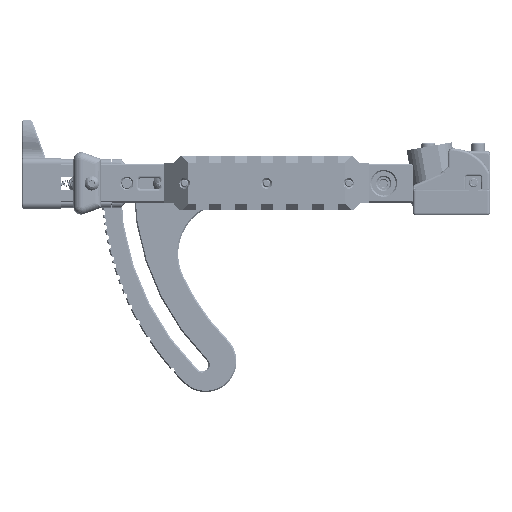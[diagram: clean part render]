
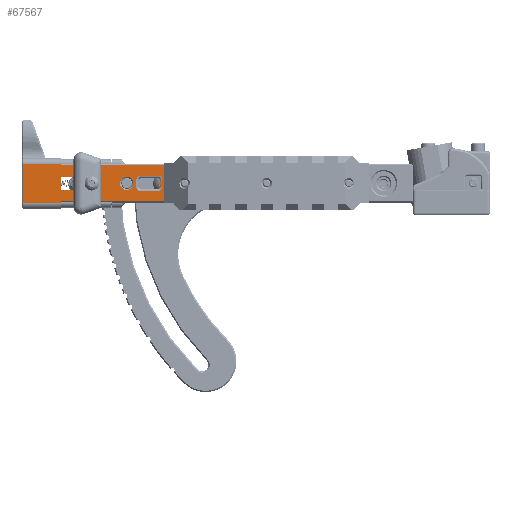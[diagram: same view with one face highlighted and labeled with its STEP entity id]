
A CAD part, left-side view. The second image highlights one B-rep face of the part: STEP entity #67567.
In plain terms, the highlighted planar face has unit normal (-1, 0, 0).
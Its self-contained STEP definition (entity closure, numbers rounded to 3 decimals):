
#2247=FACE_BOUND('',#20366,.T.);
#2248=FACE_BOUND('',#20367,.T.);
#2249=FACE_BOUND('',#20368,.T.);
#3197=PLANE('',#73201);
#6426=LINE('',#202842,#10051);
#6439=LINE('',#202868,#10064);
#6453=LINE('',#202906,#10078);
#6454=LINE('',#202908,#10079);
#6455=LINE('',#202910,#10080);
#6456=LINE('',#202912,#10081);
#6457=LINE('',#202914,#10082);
#6458=LINE('',#202915,#10083);
#6459=LINE('',#202918,#10084);
#6460=LINE('',#202920,#10085);
#6461=LINE('',#202922,#10086);
#6462=LINE('',#202923,#10087);
#6463=LINE('',#202928,#10088);
#6464=LINE('',#202930,#10089);
#6465=LINE('',#202932,#10090);
#6466=LINE('',#202936,#10091);
#6467=LINE('',#202940,#10092);
#6468=LINE('',#202944,#10093);
#6469=LINE('',#202947,#10094);
#10051=VECTOR('',#86486,10.);
#10064=VECTOR('',#86507,10.);
#10078=VECTOR('',#86529,10.);
#10079=VECTOR('',#86530,10.);
#10080=VECTOR('',#86531,10.);
#10081=VECTOR('',#86532,10.);
#10082=VECTOR('',#86533,10.);
#10083=VECTOR('',#86534,10.);
#10084=VECTOR('',#86535,10.);
#10085=VECTOR('',#86536,10.);
#10086=VECTOR('',#86537,10.);
#10087=VECTOR('',#86538,10.);
#10088=VECTOR('',#86541,10.);
#10089=VECTOR('',#86542,10.);
#10090=VECTOR('',#86543,10.);
#10091=VECTOR('',#86546,10.);
#10092=VECTOR('',#86549,10.);
#10093=VECTOR('',#86552,10.);
#10094=VECTOR('',#86555,10.);
#16200=FACE_OUTER_BOUND('',#20365,.T.);
#20365=EDGE_LOOP('',(#60392,#60393,#60394,#60395,#60396,#60397,#60398,#60399));
#20366=EDGE_LOOP('',(#60400,#60401,#60402,#60403));
#20367=EDGE_LOOP('',(#60404));
#20368=EDGE_LOOP('',(#60405,#60406,#60407,#60408,#60409,#60410,#60411,#60412,
#60413,#60414,#60415));
#22561=CIRCLE('',#73202,2.6);
#22562=CIRCLE('',#73203,1.5);
#22563=CIRCLE('',#73204,1.5);
#22564=CIRCLE('',#73205,1.5);
#22565=CIRCLE('',#73206,1.5);
#31905=VERTEX_POINT('',#202839);
#31906=VERTEX_POINT('',#202841);
#31915=VERTEX_POINT('',#202867);
#31928=VERTEX_POINT('',#202905);
#31929=VERTEX_POINT('',#202907);
#31930=VERTEX_POINT('',#202909);
#31931=VERTEX_POINT('',#202911);
#31932=VERTEX_POINT('',#202913);
#31933=VERTEX_POINT('',#202916);
#31934=VERTEX_POINT('',#202917);
#31935=VERTEX_POINT('',#202919);
#31936=VERTEX_POINT('',#202921);
#31937=VERTEX_POINT('',#202924);
#31938=VERTEX_POINT('',#202926);
#31939=VERTEX_POINT('',#202927);
#31940=VERTEX_POINT('',#202929);
#31941=VERTEX_POINT('',#202931);
#31942=VERTEX_POINT('',#202933);
#31943=VERTEX_POINT('',#202935);
#31944=VERTEX_POINT('',#202937);
#31945=VERTEX_POINT('',#202939);
#31946=VERTEX_POINT('',#202941);
#31947=VERTEX_POINT('',#202943);
#31948=VERTEX_POINT('',#202945);
#41588=EDGE_CURVE('',#31906,#31905,#6426,.T.);
#41601=EDGE_CURVE('',#31906,#31915,#6439,.T.);
#41617=EDGE_CURVE('',#31928,#31905,#6453,.T.);
#41618=EDGE_CURVE('',#31929,#31928,#6454,.T.);
#41619=EDGE_CURVE('',#31929,#31930,#6455,.T.);
#41620=EDGE_CURVE('',#31931,#31930,#6456,.T.);
#41621=EDGE_CURVE('',#31931,#31932,#6457,.T.);
#41622=EDGE_CURVE('',#31915,#31932,#6458,.T.);
#41623=EDGE_CURVE('',#31933,#31934,#6459,.T.);
#41624=EDGE_CURVE('',#31935,#31933,#6460,.T.);
#41625=EDGE_CURVE('',#31936,#31935,#6461,.T.);
#41626=EDGE_CURVE('',#31934,#31936,#6462,.T.);
#41627=EDGE_CURVE('',#31937,#31937,#22561,.T.);
#41628=EDGE_CURVE('',#31938,#31939,#6463,.T.);
#41629=EDGE_CURVE('',#31939,#31940,#6464,.T.);
#41630=EDGE_CURVE('',#31941,#31940,#6465,.T.);
#41631=EDGE_CURVE('',#31942,#31941,#22562,.T.);
#41632=EDGE_CURVE('',#31943,#31942,#6466,.T.);
#41633=EDGE_CURVE('',#31944,#31943,#22563,.T.);
#41634=EDGE_CURVE('',#31945,#31944,#6467,.T.);
#41635=EDGE_CURVE('',#31946,#31945,#22564,.T.);
#41636=EDGE_CURVE('',#31947,#31946,#6468,.T.);
#41637=EDGE_CURVE('',#31948,#31947,#22565,.T.);
#41638=EDGE_CURVE('',#31938,#31948,#6469,.T.);
#60392=ORIENTED_EDGE('',*,*,#41588,.T.);
#60393=ORIENTED_EDGE('',*,*,#41617,.F.);
#60394=ORIENTED_EDGE('',*,*,#41618,.F.);
#60395=ORIENTED_EDGE('',*,*,#41619,.T.);
#60396=ORIENTED_EDGE('',*,*,#41620,.F.);
#60397=ORIENTED_EDGE('',*,*,#41621,.T.);
#60398=ORIENTED_EDGE('',*,*,#41622,.F.);
#60399=ORIENTED_EDGE('',*,*,#41601,.F.);
#60400=ORIENTED_EDGE('',*,*,#41623,.F.);
#60401=ORIENTED_EDGE('',*,*,#41624,.F.);
#60402=ORIENTED_EDGE('',*,*,#41625,.F.);
#60403=ORIENTED_EDGE('',*,*,#41626,.F.);
#60404=ORIENTED_EDGE('',*,*,#41627,.F.);
#60405=ORIENTED_EDGE('',*,*,#41628,.T.);
#60406=ORIENTED_EDGE('',*,*,#41629,.T.);
#60407=ORIENTED_EDGE('',*,*,#41630,.F.);
#60408=ORIENTED_EDGE('',*,*,#41631,.F.);
#60409=ORIENTED_EDGE('',*,*,#41632,.F.);
#60410=ORIENTED_EDGE('',*,*,#41633,.F.);
#60411=ORIENTED_EDGE('',*,*,#41634,.F.);
#60412=ORIENTED_EDGE('',*,*,#41635,.F.);
#60413=ORIENTED_EDGE('',*,*,#41636,.F.);
#60414=ORIENTED_EDGE('',*,*,#41637,.F.);
#60415=ORIENTED_EDGE('',*,*,#41638,.F.);
#67567=ADVANCED_FACE('',(#16200,#2247,#2248,#2249),#3197,.T.);
#73201=AXIS2_PLACEMENT_3D('',#202904,#86527,#86528);
#73202=AXIS2_PLACEMENT_3D('',#202925,#86539,#86540);
#73203=AXIS2_PLACEMENT_3D('',#202934,#86544,#86545);
#73204=AXIS2_PLACEMENT_3D('',#202938,#86547,#86548);
#73205=AXIS2_PLACEMENT_3D('',#202942,#86550,#86551);
#73206=AXIS2_PLACEMENT_3D('',#202946,#86553,#86554);
#86486=DIRECTION('',(0.,0.,1.));
#86507=DIRECTION('',(0.,1.,0.));
#86527=DIRECTION('center_axis',(-1.,0.,
0.));
#86528=DIRECTION('ref_axis',(0.,0.,
1.));
#86529=DIRECTION('',(0.,-1.,0.));
#86530=DIRECTION('',(0.,0.,-1.));
#86531=DIRECTION('',(0.,1.,0.));
#86532=DIRECTION('',(0.,0.,1.));
#86533=DIRECTION('',(0.,-1.,0.));
#86534=DIRECTION('',(0.,0.,-1.));
#86535=DIRECTION('',(0.,0.,-1.));
#86536=DIRECTION('',(0.,1.,0.));
#86537=DIRECTION('',(0.,0.,1.));
#86538=DIRECTION('',(0.,-1.,0.));
#86539=DIRECTION('center_axis',(-1.,0.,
0.));
#86540=DIRECTION('ref_axis',(0.,0.,
1.));
#86541=DIRECTION('',(0.,0.866,-0.5));
#86542=DIRECTION('',(0.,-0.866,-0.5));
#86543=DIRECTION('',(0.,0.,1.));
#86544=DIRECTION('center_axis',(-1.,0.,
0.));
#86545=DIRECTION('ref_axis',(0.,-0.707,-0.707));
#86546=DIRECTION('',(0.,-1.,0.));
#86547=DIRECTION('center_axis',(-1.,0.,
0.));
#86548=DIRECTION('ref_axis',(0.,0.707,-0.707));
#86549=DIRECTION('',(0.,0.,-1.));
#86550=DIRECTION('center_axis',(-1.,0.,
0.));
#86551=DIRECTION('ref_axis',(0.,0.707,0.707));
#86552=DIRECTION('',(0.,1.,0.));
#86553=DIRECTION('center_axis',(-1.,0.,
0.));
#86554=DIRECTION('ref_axis',(0.,-0.707,0.707));
#86555=DIRECTION('',(0.,0.,1.));
#202839=CARTESIAN_POINT('',(-55.716,-306.888,31.511));
#202841=CARTESIAN_POINT('',(-55.716,-306.888,17.511));
#202842=CARTESIAN_POINT('',(-55.716,-306.888,20.476));
#202867=CARTESIAN_POINT('',(-55.71,-266.641,17.511));
#202868=CARTESIAN_POINT('',(-55.713,-289.093,17.511));
#202904=CARTESIAN_POINT('Origin',(-55.719,-326.593,24.511));
#202905=CARTESIAN_POINT('',(-55.71,-266.641,31.511));
#202906=CARTESIAN_POINT('',(-55.725,-364.093,31.511));
#202907=CARTESIAN_POINT('',(-55.71,-266.641,32.011));
#202908=CARTESIAN_POINT('',(-55.71,-266.641,24.511));
#202909=CARTESIAN_POINT('',(-55.707,-252.094,32.011));
#202910=CARTESIAN_POINT('',(-55.71,-266.641,32.011));
#202911=CARTESIAN_POINT('',(-55.707,-252.094,17.011));
#202912=CARTESIAN_POINT('',(-55.707,-252.094,19.511));
#202913=CARTESIAN_POINT('',(-55.71,-266.641,17.011));
#202914=CARTESIAN_POINT('',(-55.731,-401.593,17.011));
#202915=CARTESIAN_POINT('',(-55.71,-266.641,24.511));
#202916=CARTESIAN_POINT('',(-55.71,-266.641,27.111));
#202917=CARTESIAN_POINT('',(-55.71,-266.641,21.911));
#202918=CARTESIAN_POINT('',(-55.71,-266.641,24.511));
#202919=CARTESIAN_POINT('',(-55.712,-282.458,27.111));
#202920=CARTESIAN_POINT('',(-55.715,-296.617,27.111));
#202921=CARTESIAN_POINT('',(-55.712,-282.458,21.911));
#202922=CARTESIAN_POINT('',(-55.712,-282.458,24.511));
#202923=CARTESIAN_POINT('',(-55.715,-296.617,21.911));
#202924=CARTESIAN_POINT('',(-55.714,-292.417,21.897));
#202925=CARTESIAN_POINT('Origin',(-55.714,-292.417,24.497));
#202926=CARTESIAN_POINT('',(-55.716,-306.167,25.574));
#202927=CARTESIAN_POINT('',(-55.716,-304.301,24.497));
#202928=CARTESIAN_POINT('',(-55.717,-313.096,29.575));
#202929=CARTESIAN_POINT('',(-55.716,-306.167,23.42));
#202930=CARTESIAN_POINT('',(-55.717,-312.657,19.672));
#202931=CARTESIAN_POINT('',(-55.716,-306.167,22.997));
#202932=CARTESIAN_POINT('',(-55.716,-306.167,24.254));
#202933=CARTESIAN_POINT('',(-55.716,-304.667,21.497));
#202934=CARTESIAN_POINT('Origin',(-55.716,-304.667,22.997));
#202935=CARTESIAN_POINT('',(-55.715,-297.667,21.497));
#202936=CARTESIAN_POINT('',(-55.718,-315.63,21.497));
#202937=CARTESIAN_POINT('',(-55.714,-296.167,22.997));
#202938=CARTESIAN_POINT('Origin',(-55.715,-297.667,22.997));
#202939=CARTESIAN_POINT('',(-55.714,-296.167,25.997));
#202940=CARTESIAN_POINT('',(-55.714,-296.167,23.754));
#202941=CARTESIAN_POINT('',(-55.715,-297.667,27.497));
#202942=CARTESIAN_POINT('Origin',(-55.715,-297.667,25.997));
#202943=CARTESIAN_POINT('',(-55.716,-304.667,27.497));
#202944=CARTESIAN_POINT('',(-55.717,-312.13,27.497));
#202945=CARTESIAN_POINT('',(-55.716,-306.167,25.997));
#202946=CARTESIAN_POINT('Origin',(-55.716,-304.667,25.997));
#202947=CARTESIAN_POINT('',(-55.716,-306.167,25.254));
